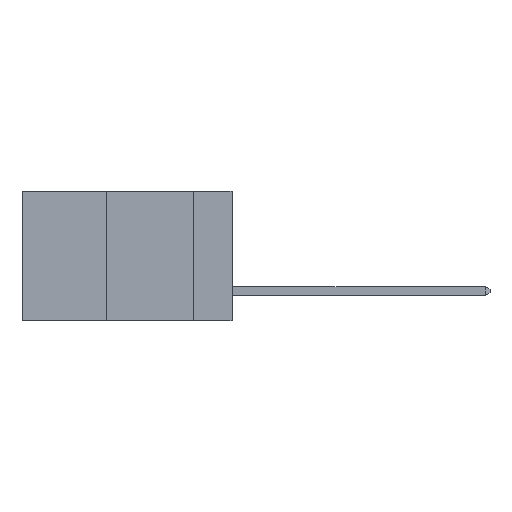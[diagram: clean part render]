
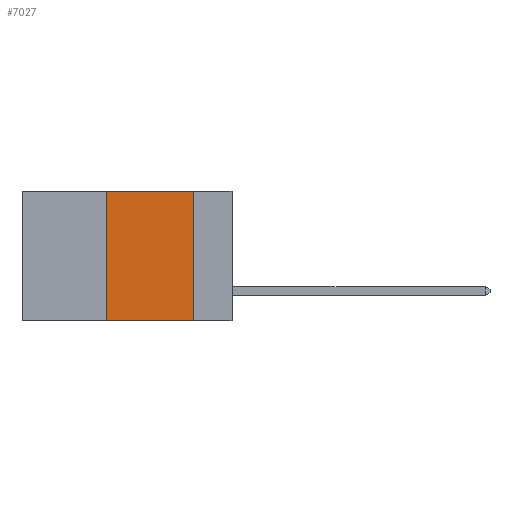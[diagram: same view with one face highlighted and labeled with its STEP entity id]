
A CAD part, left-side view. The second image highlights one B-rep face of the part: STEP entity #7027.
In plain terms, the highlighted planar face has unit normal (-1, 0, 0).
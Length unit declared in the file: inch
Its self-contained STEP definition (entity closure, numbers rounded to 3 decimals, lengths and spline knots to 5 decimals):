
#91 = CARTESIAN_POINT ( 'NONE',  ( 0., 0.36, 0. ) ) ;
#449 = DIRECTION ( 'NONE',  ( 1., 0., 0. ) ) ;
#1469 = ORIENTED_EDGE ( 'NONE', *, *, #16441, .T. ) ;
#1961 = VECTOR ( 'NONE', #13195, 39.37008 ) ;
#2035 = DIRECTION ( 'NONE',  ( 0., -1., 0. ) ) ;
#2377 = EDGE_CURVE ( 'NONE', #12086, #9162, #10877, .T. ) ;
#2495 = CARTESIAN_POINT ( 'NONE',  ( 0., 0.6, 0. ) ) ;
#2946 = EDGE_CURVE ( 'NONE', #9162, #16722, #12236, .T. ) ;
#3124 = CARTESIAN_POINT ( 'NONE',  ( 0., 0.11, 0. ) ) ;
#4653 = VECTOR ( 'NONE', #14261, 39.37008 ) ;
#5678 = LINE ( 'NONE', #10683, #1961 ) ;
#6169 = EDGE_CURVE ( 'NONE', #8518, #12086, #10169, .T. ) ;
#7027 = ADVANCED_FACE ( 'NONE', ( #13918 ), #13985, .F. ) ;
#7094 = DIRECTION ( 'NONE',  ( 0., 0., 1. ) ) ;
#7105 = CARTESIAN_POINT ( 'NONE',  ( 0., 0.36, -0.37 ) ) ;
#8518 = VERTEX_POINT ( 'NONE', #7105 ) ;
#8741 = CARTESIAN_POINT ( 'NONE',  ( 0., 0.36, 0. ) ) ;
#8803 = CARTESIAN_POINT ( 'NONE',  ( 0., 0.6, 0. ) ) ;
#9162 = VERTEX_POINT ( 'NONE', #3124 ) ;
#9806 = AXIS2_PLACEMENT_3D ( 'NONE', #8803, #449, #10226 ) ;
#10169 = LINE ( 'NONE', #91, #16530 ) ;
#10226 = DIRECTION ( 'NONE',  ( 0., 0., -1. ) ) ;
#10491 = VECTOR ( 'NONE', #2035, 39.37008 ) ;
#10683 = CARTESIAN_POINT ( 'NONE',  ( 0., 0.6, -0.37 ) ) ;
#10757 = ORIENTED_EDGE ( 'NONE', *, *, #2377, .F. ) ;
#10877 = LINE ( 'NONE', #2495, #10491 ) ;
#11952 = ORIENTED_EDGE ( 'NONE', *, *, #6169, .F. ) ;
#12086 = VERTEX_POINT ( 'NONE', #8741 ) ;
#12236 = LINE ( 'NONE', #14450, #4653 ) ;
#12903 = ORIENTED_EDGE ( 'NONE', *, *, #2946, .F. ) ;
#12969 = EDGE_LOOP ( 'NONE', ( #12903, #10757, #11952, #1469 ) ) ;
#13195 = DIRECTION ( 'NONE',  ( 0., -1., 0. ) ) ;
#13918 = FACE_OUTER_BOUND ( 'NONE', #12969, .T. ) ;
#13985 = PLANE ( 'NONE',  #9806 ) ;
#14261 = DIRECTION ( 'NONE',  ( 0., 0., -1. ) ) ;
#14450 = CARTESIAN_POINT ( 'NONE',  ( 0., 0.11, 0. ) ) ;
#15403 = CARTESIAN_POINT ( 'NONE',  ( 0., 0.11, -0.37 ) ) ;
#16441 = EDGE_CURVE ( 'NONE', #8518, #16722, #5678, .T. ) ;
#16530 = VECTOR ( 'NONE', #7094, 39.37008 ) ;
#16722 = VERTEX_POINT ( 'NONE', #15403 ) ;
